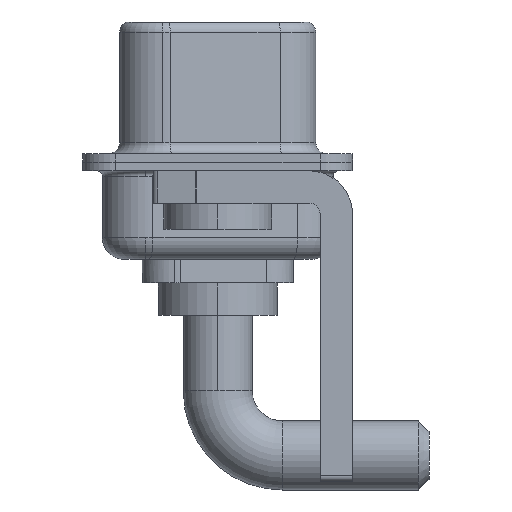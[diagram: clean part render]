
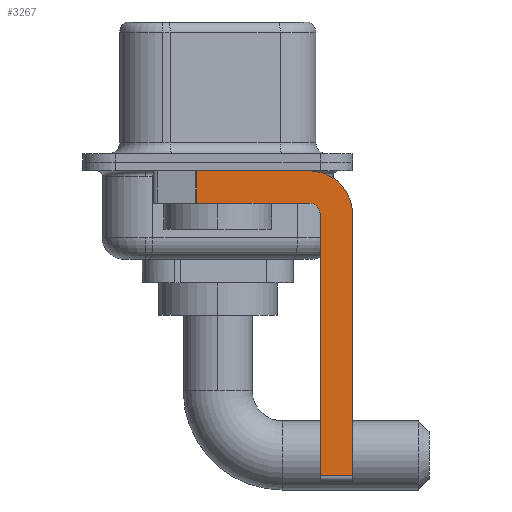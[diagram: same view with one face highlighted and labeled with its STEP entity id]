
A CAD part, left-side view. The second image highlights one B-rep face of the part: STEP entity #3267.
In plain terms, the highlighted planar face has unit normal (-1, 0, 0).
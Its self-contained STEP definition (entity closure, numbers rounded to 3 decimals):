
#143 = DIRECTION ( 'NONE',  ( 1., 0., 0. ) ) ;
#268 = VERTEX_POINT ( 'NONE', #2488 ) ;
#363 = ORIENTED_EDGE ( 'NONE', *, *, #13950, .F. ) ;
#704 = DIRECTION ( 'NONE',  ( 0., 0., 1. ) ) ;
#903 = DIRECTION ( 'NONE',  ( 0., -1., 0. ) ) ;
#1553 = VECTOR ( 'NONE', #14339, 1000. ) ;
#1954 = VERTEX_POINT ( 'NONE', #9701 ) ;
#1993 = DIRECTION ( 'NONE',  ( 1., 0., 0. ) ) ;
#2285 = CARTESIAN_POINT ( 'NONE',  ( -2.9, -4.25, -1.9 ) ) ;
#2488 = CARTESIAN_POINT ( 'NONE',  ( -2.9, -6.25, -14.55 ) ) ;
#2746 = CARTESIAN_POINT ( 'NONE',  ( -2.9, -6.25, -2.4 ) ) ;
#2852 = DIRECTION ( 'NONE',  ( 0., 0., -1. ) ) ;
#3097 = ORIENTED_EDGE ( 'NONE', *, *, #5882, .T. ) ;
#3267 = ADVANCED_FACE ( 'NONE', ( #4900 ), #3652, .F. ) ;
#3647 = ORIENTED_EDGE ( 'NONE', *, *, #13555, .F. ) ;
#3652 = PLANE ( 'NONE',  #13281 ) ;
#4160 = LINE ( 'NONE', #13159, #1553 ) ;
#4307 = CARTESIAN_POINT ( 'NONE',  ( -2.9, -4.75, -14.8 ) ) ;
#4642 = VECTOR ( 'NONE', #2852, 1000. ) ;
#4703 = CIRCLE ( 'NONE', #14123, 0.5 ) ;
#4900 = FACE_OUTER_BOUND ( 'NONE', #6440, .T. ) ;
#5083 = CARTESIAN_POINT ( 'NONE',  ( -2.9, -4.75, -2.4 ) ) ;
#5160 = DIRECTION ( 'NONE',  ( 0., 0., 1. ) ) ;
#5331 = CARTESIAN_POINT ( 'NONE',  ( -2.9, -4.25, -2.4 ) ) ;
#5667 = VERTEX_POINT ( 'NONE', #5083 ) ;
#5840 = ORIENTED_EDGE ( 'NONE', *, *, #13072, .F. ) ;
#5870 = VECTOR ( 'NONE', #903, 1000. ) ;
#5882 = EDGE_CURVE ( 'NONE', #7560, #268, #4160, .T. ) ;
#6170 = VECTOR ( 'NONE', #10162, 1000. ) ;
#6440 = EDGE_LOOP ( 'NONE', ( #7805, #15312, #363, #10433, #3647, #3097, #12742, #5840 ) ) ;
#7083 = DIRECTION ( 'NONE',  ( 0., 0., -1. ) ) ;
#7165 = VERTEX_POINT ( 'NONE', #7760 ) ;
#7188 = LINE ( 'NONE', #12659, #5870 ) ;
#7560 = VERTEX_POINT ( 'NONE', #12440 ) ;
#7760 = CARTESIAN_POINT ( 'NONE',  ( -2.9, -4.25, -0.4 ) ) ;
#7805 = ORIENTED_EDGE ( 'NONE', *, *, #8879, .F. ) ;
#8011 = DIRECTION ( 'NONE',  ( 0., 0., -1. ) ) ;
#8032 = EDGE_CURVE ( 'NONE', #8313, #1954, #11752, .T. ) ;
#8313 = VERTEX_POINT ( 'NONE', #12534 ) ;
#8879 = EDGE_CURVE ( 'NONE', #8313, #7165, #7188, .T. ) ;
#9219 = CARTESIAN_POINT ( 'NONE',  ( -2.9, 0.978, -1.9 ) ) ;
#9325 = CARTESIAN_POINT ( 'NONE',  ( -2.9, -4.25, -1.9 ) ) ;
#9404 = DIRECTION ( 'NONE',  ( 0., 1., 0. ) ) ;
#9701 = CARTESIAN_POINT ( 'NONE',  ( -2.9, 0.978, -1.9 ) ) ;
#10162 = DIRECTION ( 'NONE',  ( 0., 0., -1. ) ) ;
#10433 = ORIENTED_EDGE ( 'NONE', *, *, #16017, .F. ) ;
#10543 = VECTOR ( 'NONE', #704, 1000. ) ;
#10673 = EDGE_CURVE ( 'NONE', #14356, #268, #11440, .T. ) ;
#10720 = VERTEX_POINT ( 'NONE', #2285 ) ;
#10775 = LINE ( 'NONE', #4307, #10543 ) ;
#11057 = CIRCLE ( 'NONE', #14036, 2. ) ;
#11379 = DIRECTION ( 'NONE',  ( -1., 0., 0. ) ) ;
#11440 = LINE ( 'NONE', #16583, #6170 ) ;
#11752 = LINE ( 'NONE', #9219, #4642 ) ;
#12172 = VECTOR ( 'NONE', #9404, 1000. ) ;
#12440 = CARTESIAN_POINT ( 'NONE',  ( -2.9, -4.75, -14.55 ) ) ;
#12534 = CARTESIAN_POINT ( 'NONE',  ( -2.9, 0.978, -0.4 ) ) ;
#12659 = CARTESIAN_POINT ( 'NONE',  ( -2.9, 3., -0.4 ) ) ;
#12742 = ORIENTED_EDGE ( 'NONE', *, *, #10673, .F. ) ;
#12904 = CARTESIAN_POINT ( 'NONE',  ( -2.9, -4.25, -2.4 ) ) ;
#13072 = EDGE_CURVE ( 'NONE', #7165, #14356, #11057, .T. ) ;
#13159 = CARTESIAN_POINT ( 'NONE',  ( -2.9, -4.25, -14.55 ) ) ;
#13281 = AXIS2_PLACEMENT_3D ( 'NONE', #13510, #1993, #7083 ) ;
#13302 = LINE ( 'NONE', #9325, #12172 ) ;
#13510 = CARTESIAN_POINT ( 'NONE',  ( -2.9, -4.25, -2.4 ) ) ;
#13555 = EDGE_CURVE ( 'NONE', #7560, #5667, #10775, .T. ) ;
#13950 = EDGE_CURVE ( 'NONE', #10720, #1954, #13302, .T. ) ;
#14036 = AXIS2_PLACEMENT_3D ( 'NONE', #12904, #143, #8011 ) ;
#14123 = AXIS2_PLACEMENT_3D ( 'NONE', #5331, #11379, #5160 ) ;
#14339 = DIRECTION ( 'NONE',  ( 0., -1., 0. ) ) ;
#14356 = VERTEX_POINT ( 'NONE', #2746 ) ;
#15312 = ORIENTED_EDGE ( 'NONE', *, *, #8032, .T. ) ;
#16017 = EDGE_CURVE ( 'NONE', #5667, #10720, #4703, .T. ) ;
#16583 = CARTESIAN_POINT ( 'NONE',  ( -2.9, -6.25, -2.4 ) ) ;
